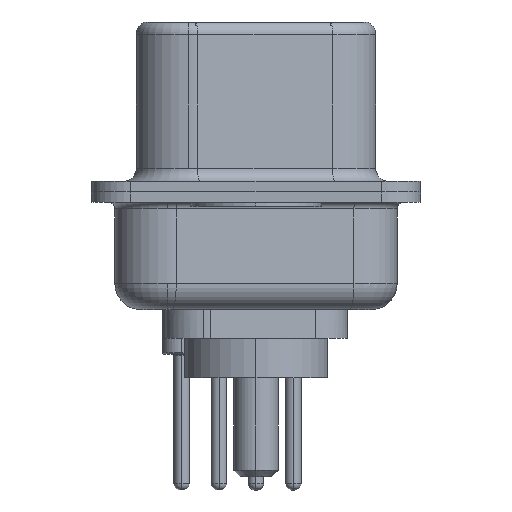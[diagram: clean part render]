
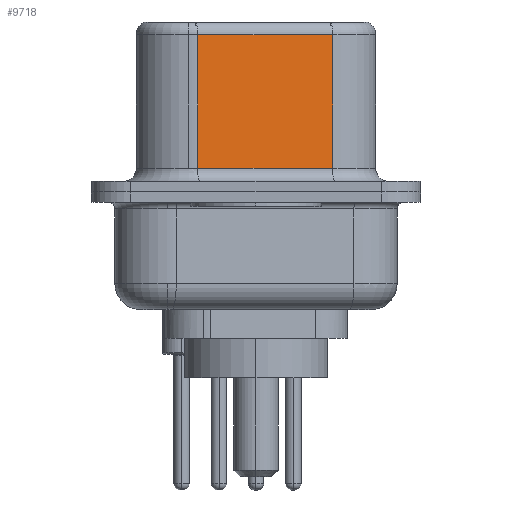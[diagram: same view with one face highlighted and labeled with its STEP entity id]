
A CAD part, left-side view. The second image highlights one B-rep face of the part: STEP entity #9718.
In plain terms, the highlighted planar face has unit normal (-0.985, -0.174, 0).
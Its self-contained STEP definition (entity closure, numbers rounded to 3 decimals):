
#1856 = VECTOR ( 'NONE', #9988, 1000. ) ;
#2392 = LINE ( 'NONE', #18933, #1856 ) ;
#2790 = EDGE_CURVE ( 'NONE', #3532, #3540, #20675, .T. ) ;
#3153 = EDGE_CURVE ( 'NONE', #15074, #19103, #18397, .T. ) ;
#3382 = CARTESIAN_POINT ( 'NONE',  ( 3.67, 2.233, 6.02 ) ) ;
#3532 = VERTEX_POINT ( 'NONE', #5076 ) ;
#3540 = VERTEX_POINT ( 'NONE', #3382 ) ;
#4158 = EDGE_CURVE ( 'NONE', #3532, #19103, #2392, .T. ) ;
#5076 = CARTESIAN_POINT ( 'NONE',  ( 4.58, -2.927, 6.02 ) ) ;
#5200 = EDGE_LOOP ( 'NONE', ( #8903, #15126, #18384, #19492 ) ) ;
#5507 = CARTESIAN_POINT ( 'NONE',  ( 3.67, 2.233, 6.52 ) ) ;
#8041 = DIRECTION ( 'NONE',  ( -0.174, 0.985, 0. ) ) ;
#8903 = ORIENTED_EDGE ( 'NONE', *, *, #4158, .F. ) ;
#9193 = EDGE_CURVE ( 'NONE', #3540, #15074, #16085, .T. ) ;
#9718 = ADVANCED_FACE ( 'NONE', ( #10901 ), #19625, .F. ) ;
#9839 = CARTESIAN_POINT ( 'NONE',  ( 4.58, -2.927, 6.52 ) ) ;
#9988 = DIRECTION ( 'NONE',  ( 0., 0., -1. ) ) ;
#10028 = DIRECTION ( 'NONE',  ( 0.985, 0.174, 0. ) ) ;
#10045 = VECTOR ( 'NONE', #12132, 1000. ) ;
#10877 = CARTESIAN_POINT ( 'NONE',  ( 4.58, -2.927, 6.02 ) ) ;
#10901 = FACE_OUTER_BOUND ( 'NONE', #5200, .T. ) ;
#12132 = DIRECTION ( 'NONE',  ( 0.174, -0.985, 0. ) ) ;
#12282 = CARTESIAN_POINT ( 'NONE',  ( 4.58, -2.927, 0.9 ) ) ;
#13771 = CARTESIAN_POINT ( 'NONE',  ( 3.67, 2.233, 0.9 ) ) ;
#15074 = VERTEX_POINT ( 'NONE', #13771 ) ;
#15126 = ORIENTED_EDGE ( 'NONE', *, *, #2790, .T. ) ;
#15167 = CARTESIAN_POINT ( 'NONE',  ( 4.58, -2.927, 0.9 ) ) ;
#16085 = LINE ( 'NONE', #5507, #16587 ) ;
#16587 = VECTOR ( 'NONE', #20186, 1000. ) ;
#17347 = DIRECTION ( 'NONE',  ( -0.174, 0.985, 0. ) ) ;
#17423 = VECTOR ( 'NONE', #8041, 1000. ) ;
#17647 = AXIS2_PLACEMENT_3D ( 'NONE', #9839, #10028, #17347 ) ;
#18384 = ORIENTED_EDGE ( 'NONE', *, *, #9193, .T. ) ;
#18397 = LINE ( 'NONE', #12282, #10045 ) ;
#18933 = CARTESIAN_POINT ( 'NONE',  ( 4.58, -2.927, 6.52 ) ) ;
#19103 = VERTEX_POINT ( 'NONE', #15167 ) ;
#19492 = ORIENTED_EDGE ( 'NONE', *, *, #3153, .T. ) ;
#19625 = PLANE ( 'NONE',  #17647 ) ;
#20186 = DIRECTION ( 'NONE',  ( 0., 0., -1. ) ) ;
#20675 = LINE ( 'NONE', #10877, #17423 ) ;
